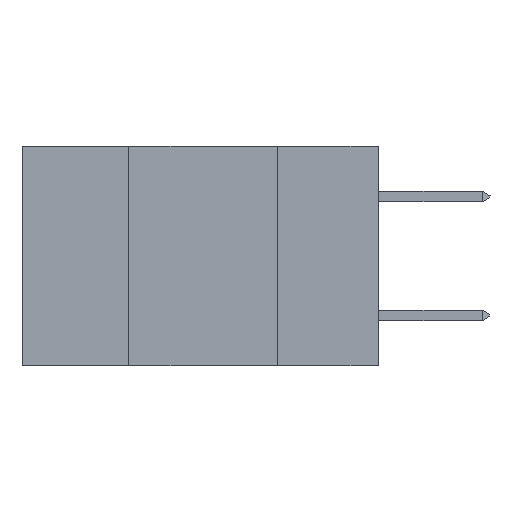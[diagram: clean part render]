
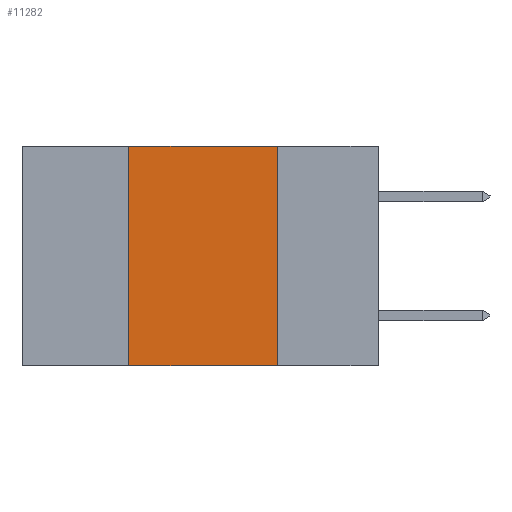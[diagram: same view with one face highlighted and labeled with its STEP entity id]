
A CAD part, left-side view. The second image highlights one B-rep face of the part: STEP entity #11282.
In plain terms, the highlighted planar face has unit normal (-1, 0, 0).
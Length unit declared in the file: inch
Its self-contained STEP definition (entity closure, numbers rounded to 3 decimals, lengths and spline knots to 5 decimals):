
#143 = VECTOR ( 'NONE', #10958, 39.37008 ) ;
#413 = LINE ( 'NONE', #9129, #143 ) ;
#420 = DIRECTION ( 'NONE',  ( 0., -1., 0. ) ) ;
#632 = ORIENTED_EDGE ( 'NONE', *, *, #11025, .F. ) ;
#1468 = EDGE_CURVE ( 'NONE', #2000, #1570, #413, .T. ) ;
#1570 = VERTEX_POINT ( 'NONE', #8050 ) ;
#2000 = VERTEX_POINT ( 'NONE', #4045 ) ;
#2147 = CARTESIAN_POINT ( 'NONE',  ( 0., 0.42, -0.37 ) ) ;
#2476 = ORIENTED_EDGE ( 'NONE', *, *, #1468, .F. ) ;
#2836 = CARTESIAN_POINT ( 'NONE',  ( 0., 0.42, -0.37 ) ) ;
#2890 = AXIS2_PLACEMENT_3D ( 'NONE', #9954, #6132, #12131 ) ;
#2914 = VERTEX_POINT ( 'NONE', #11283 ) ;
#3084 = VECTOR ( 'NONE', #8707, 39.37008 ) ;
#3824 = VECTOR ( 'NONE', #420, 39.37008 ) ;
#4045 = CARTESIAN_POINT ( 'NONE',  ( 0., 0.42, 0. ) ) ;
#4680 = LINE ( 'NONE', #2836, #3084 ) ;
#5801 = FACE_OUTER_BOUND ( 'NONE', #6727, .T. ) ;
#5827 = EDGE_CURVE ( 'NONE', #11474, #2914, #10963, .T. ) ;
#6132 = DIRECTION ( 'NONE',  ( 1., 0., 0. ) ) ;
#6542 = ORIENTED_EDGE ( 'NONE', *, *, #5827, .T. ) ;
#6727 = EDGE_LOOP ( 'NONE', ( #10162, #2476, #632, #6542 ) ) ;
#7160 = CARTESIAN_POINT ( 'NONE',  ( 0., 0.6, -0.37 ) ) ;
#8050 = CARTESIAN_POINT ( 'NONE',  ( 0., 0.17, 0. ) ) ;
#8707 = DIRECTION ( 'NONE',  ( 0., 0., 1. ) ) ;
#8961 = EDGE_CURVE ( 'NONE', #1570, #2914, #9153, .T. ) ;
#9129 = CARTESIAN_POINT ( 'NONE',  ( 0., 0.6, 0. ) ) ;
#9153 = LINE ( 'NONE', #10501, #12421 ) ;
#9697 = PLANE ( 'NONE',  #2890 ) ;
#9954 = CARTESIAN_POINT ( 'NONE',  ( 0., 0.6, 0. ) ) ;
#10162 = ORIENTED_EDGE ( 'NONE', *, *, #8961, .F. ) ;
#10501 = CARTESIAN_POINT ( 'NONE',  ( 0., 0.17, -0.37 ) ) ;
#10958 = DIRECTION ( 'NONE',  ( 0., -1., 0. ) ) ;
#10963 = LINE ( 'NONE', #7160, #3824 ) ;
#11025 = EDGE_CURVE ( 'NONE', #11474, #2000, #4680, .T. ) ;
#11282 = ADVANCED_FACE ( 'NONE', ( #5801 ), #9697, .F. ) ;
#11283 = CARTESIAN_POINT ( 'NONE',  ( 0., 0.17, -0.37 ) ) ;
#11447 = DIRECTION ( 'NONE',  ( 0., 0., -1. ) ) ;
#11474 = VERTEX_POINT ( 'NONE', #2147 ) ;
#12131 = DIRECTION ( 'NONE',  ( 0., 0., -1. ) ) ;
#12421 = VECTOR ( 'NONE', #11447, 39.37008 ) ;
